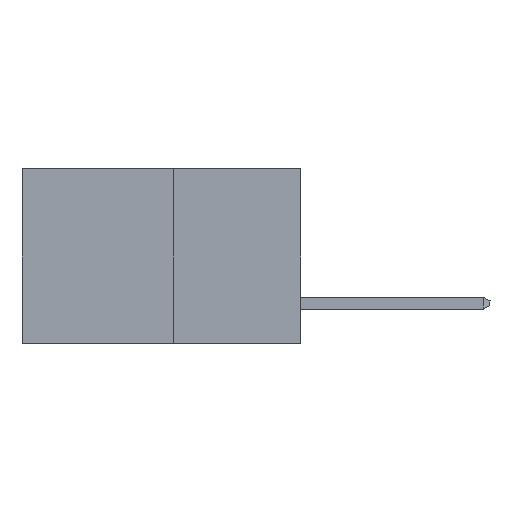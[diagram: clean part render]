
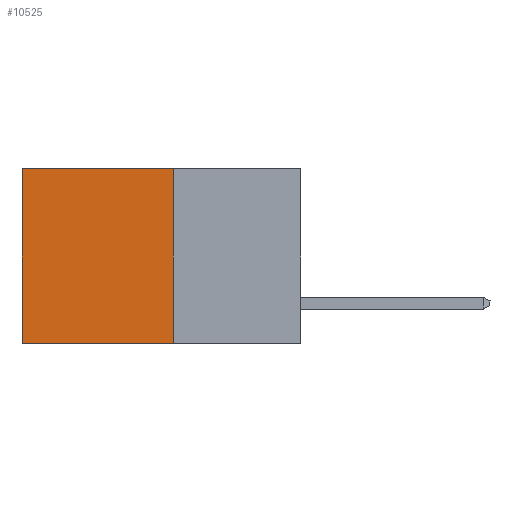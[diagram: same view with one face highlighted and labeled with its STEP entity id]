
A CAD part, left-side view. The second image highlights one B-rep face of the part: STEP entity #10525.
In plain terms, the highlighted planar face has unit normal (-1, 0, 0).
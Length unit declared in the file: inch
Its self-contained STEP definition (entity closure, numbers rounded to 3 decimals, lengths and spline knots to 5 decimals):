
#17 = DIRECTION ( 'NONE',  ( 0., 0., -1. ) ) ;
#31 = CARTESIAN_POINT ( 'NONE',  ( 0.277, 0.27, -0.37 ) ) ;
#296 = ORIENTED_EDGE ( 'NONE', *, *, #8088, .T. ) ;
#399 = ORIENTED_EDGE ( 'NONE', *, *, #5486, .F. ) ;
#417 = VERTEX_POINT ( 'NONE', #4409 ) ;
#531 = AXIS2_PLACEMENT_3D ( 'NONE', #746, #9001, #4106 ) ;
#746 = CARTESIAN_POINT ( 'NONE',  ( 0.277, 0.27, -0.37 ) ) ;
#885 = DIRECTION ( 'NONE',  ( 0., 1., 0. ) ) ;
#2934 = DIRECTION ( 'NONE',  ( 0., 0., -1. ) ) ;
#2986 = EDGE_LOOP ( 'NONE', ( #5330, #6607, #399, #296 ) ) ;
#3276 = PLANE ( 'NONE',  #531 ) ;
#3373 = CARTESIAN_POINT ( 'NONE',  ( 0.277, 0.59, -0.37 ) ) ;
#3741 = LINE ( 'NONE', #5374, #5405 ) ;
#3798 = CARTESIAN_POINT ( 'NONE',  ( 0.277, 0.27, 0. ) ) ;
#4106 = DIRECTION ( 'NONE',  ( 0., 0., -1. ) ) ;
#4281 = VECTOR ( 'NONE', #4626, 39.37008 ) ;
#4409 = CARTESIAN_POINT ( 'NONE',  ( 0.277, 0.27, 0. ) ) ;
#4626 = DIRECTION ( 'NONE',  ( 0., 1., 0. ) ) ;
#4968 = CARTESIAN_POINT ( 'NONE',  ( 0.277, 0.27, -0.37 ) ) ;
#5330 = ORIENTED_EDGE ( 'NONE', *, *, #9463, .T. ) ;
#5374 = CARTESIAN_POINT ( 'NONE',  ( 0.277, 0.27, -0.37 ) ) ;
#5405 = VECTOR ( 'NONE', #2934, 39.37008 ) ;
#5486 = EDGE_CURVE ( 'NONE', #417, #8415, #3741, .T. ) ;
#5922 = LINE ( 'NONE', #3798, #4281 ) ;
#6231 = CARTESIAN_POINT ( 'NONE',  ( 0.277, 0.59, -0.37 ) ) ;
#6607 = ORIENTED_EDGE ( 'NONE', *, *, #10608, .F. ) ;
#6845 = VERTEX_POINT ( 'NONE', #6231 ) ;
#6928 = VERTEX_POINT ( 'NONE', #8843 ) ;
#7028 = FACE_OUTER_BOUND ( 'NONE', #2986, .T. ) ;
#7183 = VECTOR ( 'NONE', #17, 39.37008 ) ;
#8088 = EDGE_CURVE ( 'NONE', #417, #6928, #5922, .T. ) ;
#8415 = VERTEX_POINT ( 'NONE', #4968 ) ;
#8843 = CARTESIAN_POINT ( 'NONE',  ( 0.277, 0.59, 0. ) ) ;
#9001 = DIRECTION ( 'NONE',  ( 1., 0., 0. ) ) ;
#9371 = LINE ( 'NONE', #3373, #7183 ) ;
#9463 = EDGE_CURVE ( 'NONE', #6928, #6845, #9371, .T. ) ;
#10102 = LINE ( 'NONE', #31, #10348 ) ;
#10348 = VECTOR ( 'NONE', #885, 39.37008 ) ;
#10525 = ADVANCED_FACE ( 'NONE', ( #7028 ), #3276, .F. ) ;
#10608 = EDGE_CURVE ( 'NONE', #8415, #6845, #10102, .T. ) ;
